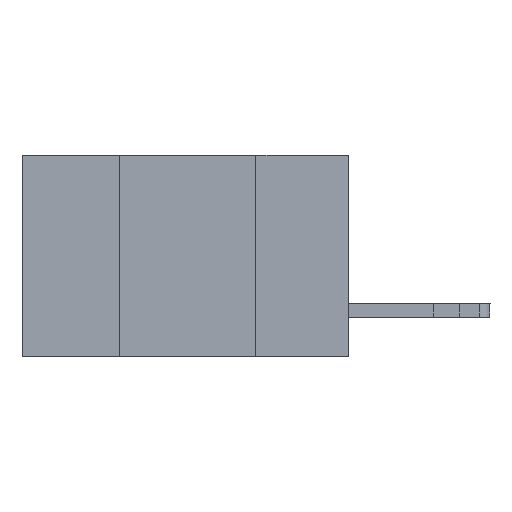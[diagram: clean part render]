
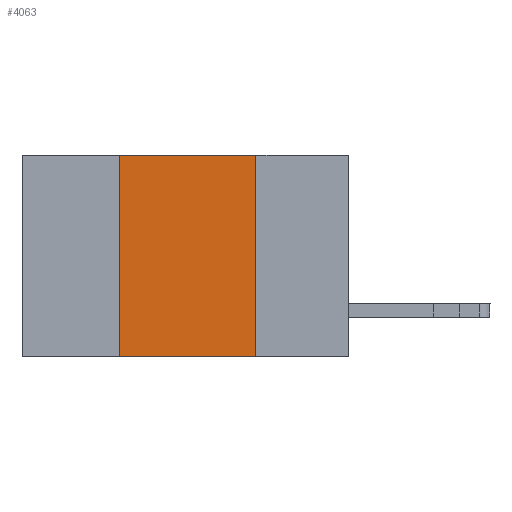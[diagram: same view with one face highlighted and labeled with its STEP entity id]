
A CAD part, left-side view. The second image highlights one B-rep face of the part: STEP entity #4063.
In plain terms, the highlighted planar face has unit normal (-1, 0, 0).
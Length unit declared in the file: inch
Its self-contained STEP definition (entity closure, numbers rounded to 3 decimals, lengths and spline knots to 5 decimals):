
#285 = LINE ( 'NONE', #5412, #13464 ) ;
#768 = EDGE_CURVE ( 'NONE', #13949, #11200, #5613, .T. ) ;
#869 = CARTESIAN_POINT ( 'NONE',  ( 0., 0.17, -0.37 ) ) ;
#1247 = DIRECTION ( 'NONE',  ( 0., 0., -1. ) ) ;
#1301 = CARTESIAN_POINT ( 'NONE',  ( 0., 0.6, 0. ) ) ;
#1589 = EDGE_CURVE ( 'NONE', #12808, #3530, #4370, .T. ) ;
#2345 = CARTESIAN_POINT ( 'NONE',  ( 0., 0.6, 0. ) ) ;
#2422 = EDGE_LOOP ( 'NONE', ( #10451, #4289, #6768, #2687 ) ) ;
#2687 = ORIENTED_EDGE ( 'NONE', *, *, #768, .T. ) ;
#3530 = VERTEX_POINT ( 'NONE', #6828 ) ;
#4063 = ADVANCED_FACE ( 'NONE', ( #6711 ), #7851, .F. ) ;
#4289 = ORIENTED_EDGE ( 'NONE', *, *, #1589, .F. ) ;
#4370 = LINE ( 'NONE', #2345, #6390 ) ;
#4536 = CARTESIAN_POINT ( 'NONE',  ( 0., 0.42, 0. ) ) ;
#4951 = CARTESIAN_POINT ( 'NONE',  ( 0., 0.17, 0. ) ) ;
#5412 = CARTESIAN_POINT ( 'NONE',  ( 0., 0.42, 0. ) ) ;
#5613 = LINE ( 'NONE', #7336, #12201 ) ;
#6390 = VECTOR ( 'NONE', #11283, 39.37008 ) ;
#6711 = FACE_OUTER_BOUND ( 'NONE', #2422, .T. ) ;
#6768 = ORIENTED_EDGE ( 'NONE', *, *, #16415, .F. ) ;
#6828 = CARTESIAN_POINT ( 'NONE',  ( 0., 0.17, 0. ) ) ;
#6916 = VECTOR ( 'NONE', #11249, 39.37008 ) ;
#7336 = CARTESIAN_POINT ( 'NONE',  ( 0., 0.6, -0.37 ) ) ;
#7851 = PLANE ( 'NONE',  #11914 ) ;
#7907 = LINE ( 'NONE', #4951, #6916 ) ;
#8743 = CARTESIAN_POINT ( 'NONE',  ( 0., 0.42, -0.37 ) ) ;
#8782 = EDGE_CURVE ( 'NONE', #3530, #11200, #7907, .T. ) ;
#9915 = DIRECTION ( 'NONE',  ( 0., -1., 0. ) ) ;
#10451 = ORIENTED_EDGE ( 'NONE', *, *, #8782, .F. ) ;
#11200 = VERTEX_POINT ( 'NONE', #869 ) ;
#11249 = DIRECTION ( 'NONE',  ( 0., 0., -1. ) ) ;
#11283 = DIRECTION ( 'NONE',  ( 0., -1., 0. ) ) ;
#11686 = DIRECTION ( 'NONE',  ( 1., 0., 0. ) ) ;
#11914 = AXIS2_PLACEMENT_3D ( 'NONE', #1301, #11686, #1247 ) ;
#12201 = VECTOR ( 'NONE', #9915, 39.37008 ) ;
#12808 = VERTEX_POINT ( 'NONE', #4536 ) ;
#13464 = VECTOR ( 'NONE', #15638, 39.37008 ) ;
#13949 = VERTEX_POINT ( 'NONE', #8743 ) ;
#15638 = DIRECTION ( 'NONE',  ( 0., 0., 1. ) ) ;
#16415 = EDGE_CURVE ( 'NONE', #13949, #12808, #285, .T. ) ;
